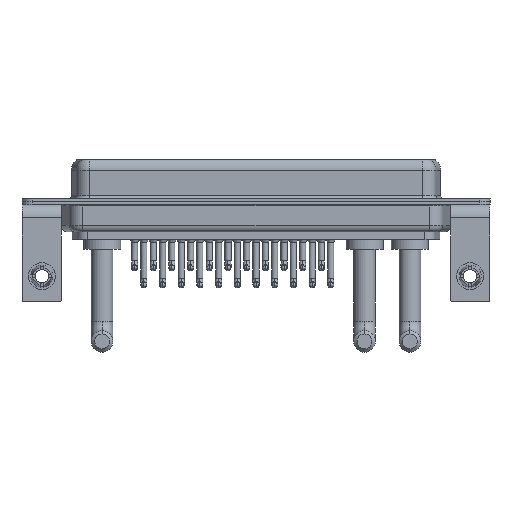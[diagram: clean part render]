
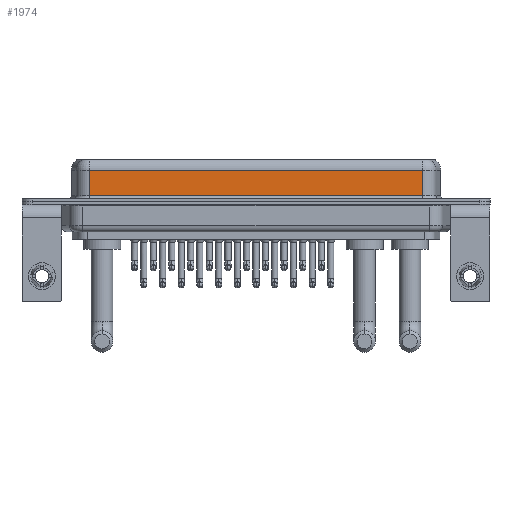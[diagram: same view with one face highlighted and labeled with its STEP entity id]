
A CAD part, front view. The second image highlights one B-rep face of the part: STEP entity #1974.
In plain terms, the highlighted planar face has unit normal (0, -1, 0).
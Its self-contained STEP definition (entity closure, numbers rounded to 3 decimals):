
#1284 = DIRECTION ( 'NONE',  ( 0., 0., 1. ) ) ;
#1446 = VERTEX_POINT ( 'NONE', #9319 ) ;
#1803 = VERTEX_POINT ( 'NONE', #18935 ) ;
#1974 = ADVANCED_FACE ( 'NONE', ( #13367 ), #25522, .F. ) ;
#2655 = ORIENTED_EDGE ( 'NONE', *, *, #11198, .T. ) ;
#2749 = LINE ( 'NONE', #15075, #20430 ) ;
#2770 = VECTOR ( 'NONE', #22941, 1000. ) ;
#3024 = CARTESIAN_POINT ( 'NONE',  ( 56.462, -3.95, 6.4 ) ) ;
#3851 = VECTOR ( 'NONE', #13445, 1000. ) ;
#4007 = ORIENTED_EDGE ( 'NONE', *, *, #24678, .F. ) ;
#5345 = CARTESIAN_POINT ( 'NONE',  ( 56.462, -3.95, 4.65 ) ) ;
#5887 = VECTOR ( 'NONE', #22289, 1000. ) ;
#6128 = LINE ( 'NONE', #14220, #5887 ) ;
#6182 = VERTEX_POINT ( 'NONE', #18331 ) ;
#6314 = EDGE_CURVE ( 'NONE', #26124, #1803, #6128, .T. ) ;
#7399 = DIRECTION ( 'NONE',  ( 0., 1., 0. ) ) ;
#9319 = CARTESIAN_POINT ( 'NONE',  ( 56.462, -3.95, 4.65 ) ) ;
#11032 = ORIENTED_EDGE ( 'NONE', *, *, #6314, .T. ) ;
#11198 = EDGE_CURVE ( 'NONE', #6182, #26124, #15000, .T. ) ;
#13096 = DIRECTION ( 'NONE',  ( 0., 0., -1. ) ) ;
#13367 = FACE_OUTER_BOUND ( 'NONE', #17202, .T. ) ;
#13445 = DIRECTION ( 'NONE',  ( -1., 0., 0. ) ) ;
#14220 = CARTESIAN_POINT ( 'NONE',  ( 56.462, -3.95, 0.9 ) ) ;
#14442 = AXIS2_PLACEMENT_3D ( 'NONE', #3024, #7399, #1284 ) ;
#15000 = LINE ( 'NONE', #20818, #2770 ) ;
#15075 = CARTESIAN_POINT ( 'NONE',  ( 56.462, -3.95, 6.4 ) ) ;
#15316 = LINE ( 'NONE', #5345, #3851 ) ;
#17202 = EDGE_LOOP ( 'NONE', ( #4007, #17229, #2655, #11032 ) ) ;
#17229 = ORIENTED_EDGE ( 'NONE', *, *, #23362, .T. ) ;
#18331 = CARTESIAN_POINT ( 'NONE',  ( 7.038, -3.95, 4.65 ) ) ;
#18935 = CARTESIAN_POINT ( 'NONE',  ( 56.462, -3.95, 0.9 ) ) ;
#20430 = VECTOR ( 'NONE', #13096, 1000. ) ;
#20818 = CARTESIAN_POINT ( 'NONE',  ( 7.038, -3.95, 6.4 ) ) ;
#22289 = DIRECTION ( 'NONE',  ( 1., 0., 0. ) ) ;
#22504 = CARTESIAN_POINT ( 'NONE',  ( 7.038, -3.95, 0.9 ) ) ;
#22941 = DIRECTION ( 'NONE',  ( 0., 0., -1. ) ) ;
#23362 = EDGE_CURVE ( 'NONE', #1446, #6182, #15316, .T. ) ;
#24678 = EDGE_CURVE ( 'NONE', #1446, #1803, #2749, .T. ) ;
#25522 = PLANE ( 'NONE',  #14442 ) ;
#26124 = VERTEX_POINT ( 'NONE', #22504 ) ;
